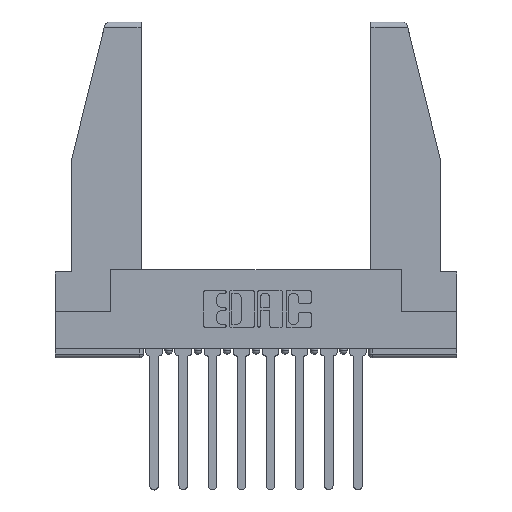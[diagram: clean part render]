
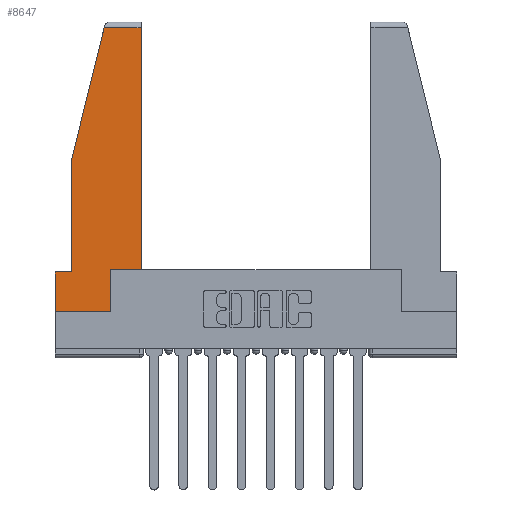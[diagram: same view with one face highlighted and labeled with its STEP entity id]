
A CAD part, top view. The second image highlights one B-rep face of the part: STEP entity #8647.
In plain terms, the highlighted planar face has unit normal (0, 0, 1).
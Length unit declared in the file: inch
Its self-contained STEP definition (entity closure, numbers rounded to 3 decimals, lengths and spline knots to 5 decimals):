
#7 = CARTESIAN_POINT ( 'NONE',  ( 0.461, 0.223, 0. ) ) ;
#10 = DIRECTION ( 'NONE',  ( -0.239, -0.971, 0. ) ) ;
#36 = VERTEX_POINT ( 'NONE', #11407 ) ;
#76 = VERTEX_POINT ( 'NONE', #1311 ) ;
#139 = DIRECTION ( 'NONE',  ( 0., -1., 0. ) ) ;
#357 = CARTESIAN_POINT ( 'NONE',  ( 0.297, 0., 0. ) ) ;
#410 = VECTOR ( 'NONE', #4491, 39.37008 ) ;
#670 = LINE ( 'NONE', #2295, #11768 ) ;
#727 = CARTESIAN_POINT ( 'NONE',  ( 0.297, 0.223, 0. ) ) ;
#1228 = EDGE_CURVE ( 'NONE', #11277, #36, #4239, .T. ) ;
#1306 = LINE ( 'NONE', #2356, #11596 ) ;
#1311 = CARTESIAN_POINT ( 'NONE',  ( 0.2636, 1.52, 0. ) ) ;
#1459 = VERTEX_POINT ( 'NONE', #7 ) ;
#1799 = ORIENTED_EDGE ( 'NONE', *, *, #10341, .T. ) ;
#1838 = VERTEX_POINT ( 'NONE', #7382 ) ;
#1915 = EDGE_CURVE ( 'NONE', #13063, #3143, #1306, .T. ) ;
#2267 = EDGE_CURVE ( 'NONE', #36, #13063, #12224, .T. ) ;
#2295 = CARTESIAN_POINT ( 'NONE',  ( 0.271, 1.55, 0. ) ) ;
#2296 = DIRECTION ( 'NONE',  ( -1., 0., 0. ) ) ;
#2356 = CARTESIAN_POINT ( 'NONE',  ( 0., 0., 0. ) ) ;
#3143 = VERTEX_POINT ( 'NONE', #11867 ) ;
#3743 = EDGE_CURVE ( 'NONE', #1459, #1838, #9826, .T. ) ;
#4239 = LINE ( 'NONE', #11109, #8798 ) ;
#4294 = EDGE_LOOP ( 'NONE', ( #12632, #8502, #6799, #11122, #11456, #4592, #7312, #9153, #1799 ) ) ;
#4308 = CARTESIAN_POINT ( 'NONE',  ( 0., 0., 0. ) ) ;
#4327 = EDGE_CURVE ( 'NONE', #76, #11949, #670, .T. ) ;
#4491 = DIRECTION ( 'NONE',  ( 0., -1., 0. ) ) ;
#4537 = CARTESIAN_POINT ( 'NONE',  ( 0.086, 0.8, 0. ) ) ;
#4592 = ORIENTED_EDGE ( 'NONE', *, *, #2267, .T. ) ;
#4823 = CARTESIAN_POINT ( 'NONE',  ( 0.297, 0.223, 0. ) ) ;
#6322 = CARTESIAN_POINT ( 'NONE',  ( 0.086, 0.21, 0. ) ) ;
#6455 = LINE ( 'NONE', #11689, #10078 ) ;
#6799 = ORIENTED_EDGE ( 'NONE', *, *, #4327, .T. ) ;
#6889 = VECTOR ( 'NONE', #7558, 39.37008 ) ;
#7312 = ORIENTED_EDGE ( 'NONE', *, *, #1915, .T. ) ;
#7382 = CARTESIAN_POINT ( 'NONE',  ( 0.461, 1.52, 0. ) ) ;
#7558 = DIRECTION ( 'NONE',  ( 0., 1., 0. ) ) ;
#7670 = VECTOR ( 'NONE', #8563, 39.37008 ) ;
#7709 = LINE ( 'NONE', #4537, #410 ) ;
#8064 = DIRECTION ( 'NONE',  ( -1., 0., 0. ) ) ;
#8361 = VERTEX_POINT ( 'NONE', #4823 ) ;
#8502 = ORIENTED_EDGE ( 'NONE', *, *, #9316, .T. ) ;
#8563 = DIRECTION ( 'NONE',  ( 0., 1., 0. ) ) ;
#8647 = ADVANCED_FACE ( 'NONE', ( #11820 ), #10549, .T. ) ;
#8733 = EDGE_CURVE ( 'NONE', #3143, #8361, #9868, .T. ) ;
#8798 = VECTOR ( 'NONE', #8064, 39.37008 ) ;
#9153 = ORIENTED_EDGE ( 'NONE', *, *, #8733, .T. ) ;
#9316 = EDGE_CURVE ( 'NONE', #1838, #76, #6455, .T. ) ;
#9639 = CARTESIAN_POINT ( 'NONE',  ( 0.461, 0.223, 0. ) ) ;
#9656 = DIRECTION ( 'NONE',  ( 1., 0., 0. ) ) ;
#9826 = LINE ( 'NONE', #9639, #7670 ) ;
#9868 = LINE ( 'NONE', #357, #6889 ) ;
#10078 = VECTOR ( 'NONE', #2296, 39.37008 ) ;
#10341 = EDGE_CURVE ( 'NONE', #8361, #1459, #13125, .T. ) ;
#10549 = PLANE ( 'NONE',  #11211 ) ;
#11047 = VECTOR ( 'NONE', #13038, 39.37008 ) ;
#11109 = CARTESIAN_POINT ( 'NONE',  ( 0., 0.21, 0. ) ) ;
#11122 = ORIENTED_EDGE ( 'NONE', *, *, #11984, .T. ) ;
#11211 = AXIS2_PLACEMENT_3D ( 'NONE', #4308, #11622, #12638 ) ;
#11277 = VERTEX_POINT ( 'NONE', #6322 ) ;
#11407 = CARTESIAN_POINT ( 'NONE',  ( 0., 0.21, 0. ) ) ;
#11456 = ORIENTED_EDGE ( 'NONE', *, *, #1228, .T. ) ;
#11476 = CARTESIAN_POINT ( 'NONE',  ( 0., 0., 0. ) ) ;
#11596 = VECTOR ( 'NONE', #9656, 39.37008 ) ;
#11622 = DIRECTION ( 'NONE',  ( 0., 0., 1. ) ) ;
#11689 = CARTESIAN_POINT ( 'NONE',  ( 0., 1.52, 0. ) ) ;
#11768 = VECTOR ( 'NONE', #10, 39.37008 ) ;
#11820 = FACE_OUTER_BOUND ( 'NONE', #4294, .T. ) ;
#11867 = CARTESIAN_POINT ( 'NONE',  ( 0.297, 0., 0. ) ) ;
#11895 = CARTESIAN_POINT ( 'NONE',  ( 0.086, 0.8, 0. ) ) ;
#11949 = VERTEX_POINT ( 'NONE', #11895 ) ;
#11984 = EDGE_CURVE ( 'NONE', #11949, #11277, #7709, .T. ) ;
#12224 = LINE ( 'NONE', #12611, #13159 ) ;
#12611 = CARTESIAN_POINT ( 'NONE',  ( 0., 0.21, 0. ) ) ;
#12632 = ORIENTED_EDGE ( 'NONE', *, *, #3743, .T. ) ;
#12638 = DIRECTION ( 'NONE',  ( 1., 0., 0. ) ) ;
#13038 = DIRECTION ( 'NONE',  ( 1., 0., 0. ) ) ;
#13063 = VERTEX_POINT ( 'NONE', #11476 ) ;
#13125 = LINE ( 'NONE', #727, #11047 ) ;
#13159 = VECTOR ( 'NONE', #139, 39.37008 ) ;
